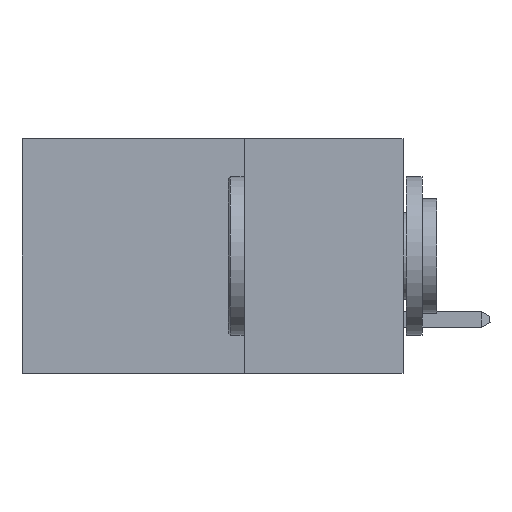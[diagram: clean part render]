
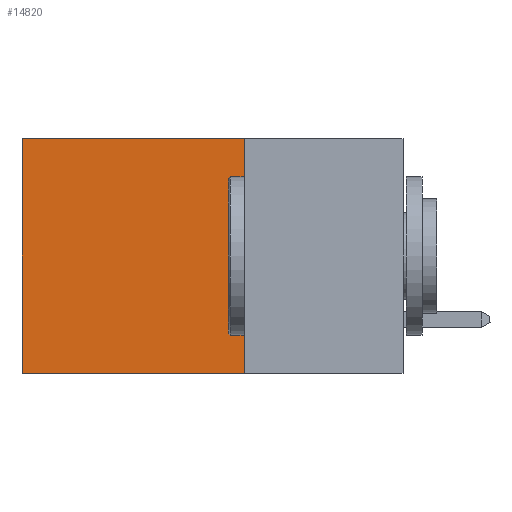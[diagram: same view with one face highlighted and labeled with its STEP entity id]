
A CAD part, left-side view. The second image highlights one B-rep face of the part: STEP entity #14820.
In plain terms, the highlighted planar face has unit normal (-1, 0, 0).
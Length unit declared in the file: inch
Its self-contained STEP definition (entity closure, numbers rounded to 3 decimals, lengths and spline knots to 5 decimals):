
#1054 = EDGE_LOOP ( 'NONE', ( #9351, #33756, #10818, #35207 ) ) ;
#2487 = DIRECTION ( 'NONE',  ( 1., 0., 0. ) ) ;
#3454 = VECTOR ( 'NONE', #32559, 39.37008 ) ;
#3584 = CARTESIAN_POINT ( 'NONE',  ( 0.2875, 0.25, 0. ) ) ;
#3869 = VERTEX_POINT ( 'NONE', #3584 ) ;
#5725 = VERTEX_POINT ( 'NONE', #22510 ) ;
#6961 = AXIS2_PLACEMENT_3D ( 'NONE', #20105, #2487, #23070 ) ;
#8532 = VECTOR ( 'NONE', #14138, 39.37008 ) ;
#9200 = CARTESIAN_POINT ( 'NONE',  ( 0.2875, 0.25, 0. ) ) ;
#9351 = ORIENTED_EDGE ( 'NONE', *, *, #30872, .T. ) ;
#10033 = VECTOR ( 'NONE', #33531, 39.37008 ) ;
#10192 = CARTESIAN_POINT ( 'NONE',  ( 0.2875, 0.25, 0. ) ) ;
#10818 = ORIENTED_EDGE ( 'NONE', *, *, #35547, .F. ) ;
#12230 = LINE ( 'NONE', #9200, #3454 ) ;
#14138 = DIRECTION ( 'NONE',  ( 0., 1., 0. ) ) ;
#14820 = ADVANCED_FACE ( 'NONE', ( #27503 ), #17132, .F. ) ;
#15726 = CARTESIAN_POINT ( 'NONE',  ( 0.2875, 0.6, 0. ) ) ;
#17132 = PLANE ( 'NONE',  #6961 ) ;
#18564 = LINE ( 'NONE', #19803, #24540 ) ;
#18937 = VERTEX_POINT ( 'NONE', #15726 ) ;
#19803 = CARTESIAN_POINT ( 'NONE',  ( 0.2875, 0.6, 0. ) ) ;
#20105 = CARTESIAN_POINT ( 'NONE',  ( 0.2875, 0.25, 0. ) ) ;
#22510 = CARTESIAN_POINT ( 'NONE',  ( 0.2875, 0.25, -0.37 ) ) ;
#23070 = DIRECTION ( 'NONE',  ( 0., 0., -1. ) ) ;
#24540 = VECTOR ( 'NONE', #25555, 39.37008 ) ;
#25555 = DIRECTION ( 'NONE',  ( 0., 0., -1. ) ) ;
#25604 = LINE ( 'NONE', #10192, #10033 ) ;
#26362 = EDGE_CURVE ( 'NONE', #3869, #18937, #25604, .T. ) ;
#27503 = FACE_OUTER_BOUND ( 'NONE', #1054, .T. ) ;
#27668 = CARTESIAN_POINT ( 'NONE',  ( 0.2875, 0.6, -0.37 ) ) ;
#28529 = EDGE_CURVE ( 'NONE', #5725, #29427, #31797, .T. ) ;
#29427 = VERTEX_POINT ( 'NONE', #27668 ) ;
#30872 = EDGE_CURVE ( 'NONE', #18937, #29427, #18564, .T. ) ;
#31570 = CARTESIAN_POINT ( 'NONE',  ( 0.2875, 0.25, -0.37 ) ) ;
#31797 = LINE ( 'NONE', #31570, #8532 ) ;
#32559 = DIRECTION ( 'NONE',  ( 0., 0., -1. ) ) ;
#33531 = DIRECTION ( 'NONE',  ( 0., 1., 0. ) ) ;
#33756 = ORIENTED_EDGE ( 'NONE', *, *, #28529, .F. ) ;
#35207 = ORIENTED_EDGE ( 'NONE', *, *, #26362, .T. ) ;
#35547 = EDGE_CURVE ( 'NONE', #3869, #5725, #12230, .T. ) ;
